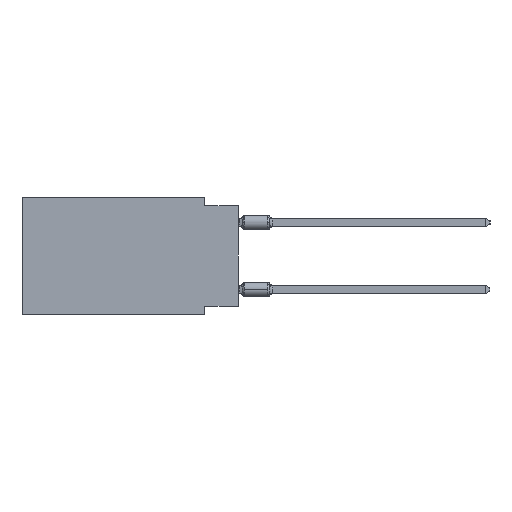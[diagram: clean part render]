
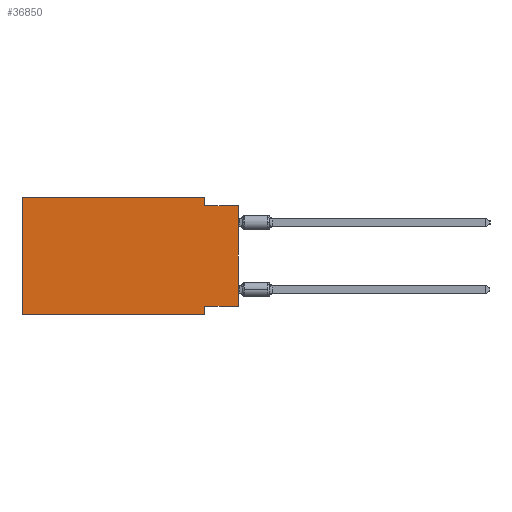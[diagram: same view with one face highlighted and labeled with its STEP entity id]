
A CAD part, left-side view. The second image highlights one B-rep face of the part: STEP entity #36850.
In plain terms, the highlighted planar face has unit normal (-1, 0, 0).
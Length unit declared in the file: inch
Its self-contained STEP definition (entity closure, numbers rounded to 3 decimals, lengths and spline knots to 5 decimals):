
#1203 = CARTESIAN_POINT ( 'NONE',  ( 0., 0., -0.025 ) ) ;
#2034 = ORIENTED_EDGE ( 'NONE', *, *, #37414, .F. ) ;
#2503 = EDGE_CURVE ( 'NONE', #30839, #32852, #24067, .T. ) ;
#3058 = DIRECTION ( 'NONE',  ( 0., -1., 0. ) ) ;
#3201 = EDGE_CURVE ( 'NONE', #14158, #42809, #20255, .T. ) ;
#3870 = DIRECTION ( 'NONE',  ( 0., 0., 1. ) ) ;
#6277 = ORIENTED_EDGE ( 'NONE', *, *, #2503, .F. ) ;
#7036 = VECTOR ( 'NONE', #18807, 39.37008 ) ;
#7081 = EDGE_CURVE ( 'NONE', #27757, #14158, #14231, .T. ) ;
#7306 = LINE ( 'NONE', #21263, #9788 ) ;
#7360 = EDGE_CURVE ( 'NONE', #15903, #43868, #16924, .T. ) ;
#7708 = LINE ( 'NONE', #42487, #31063 ) ;
#9788 = VECTOR ( 'NONE', #3870, 39.37008 ) ;
#9814 = CARTESIAN_POINT ( 'NONE',  ( 0., 0.645, -0.35 ) ) ;
#10117 = FACE_OUTER_BOUND ( 'NONE', #29956, .T. ) ;
#11019 = CARTESIAN_POINT ( 'NONE',  ( 0., 0.1, 0. ) ) ;
#11579 = ORIENTED_EDGE ( 'NONE', *, *, #42791, .F. ) ;
#11835 = EDGE_CURVE ( 'NONE', #30839, #42809, #7708, .T. ) ;
#12063 = CARTESIAN_POINT ( 'NONE',  ( 0., 0.1, 0. ) ) ;
#12819 = AXIS2_PLACEMENT_3D ( 'NONE', #44896, #41465, #17667 ) ;
#13670 = DIRECTION ( 'NONE',  ( 0., 0., 1. ) ) ;
#14158 = VERTEX_POINT ( 'NONE', #15930 ) ;
#14231 = LINE ( 'NONE', #11019, #20646 ) ;
#15883 = VECTOR ( 'NONE', #40990, 39.37008 ) ;
#15903 = VERTEX_POINT ( 'NONE', #40662 ) ;
#15930 = CARTESIAN_POINT ( 'NONE',  ( 0., 0.1, -0.025 ) ) ;
#16818 = CARTESIAN_POINT ( 'NONE',  ( 0., 0., -0.025 ) ) ;
#16907 = VERTEX_POINT ( 'NONE', #29260 ) ;
#16924 = LINE ( 'NONE', #9814, #40402 ) ;
#17667 = DIRECTION ( 'NONE',  ( 0., 0., -1. ) ) ;
#18807 = DIRECTION ( 'NONE',  ( 0., 0., -1. ) ) ;
#20255 = LINE ( 'NONE', #16818, #44344 ) ;
#20548 = ORIENTED_EDGE ( 'NONE', *, *, #3201, .F. ) ;
#20646 = VECTOR ( 'NONE', #38940, 39.37008 ) ;
#21263 = CARTESIAN_POINT ( 'NONE',  ( 0., 0.645, 0. ) ) ;
#21306 = ORIENTED_EDGE ( 'NONE', *, *, #31926, .F. ) ;
#22227 = CARTESIAN_POINT ( 'NONE',  ( 0., 0.1, -0.35 ) ) ;
#23653 = LINE ( 'NONE', #37848, #30740 ) ;
#23673 = DIRECTION ( 'NONE',  ( 0., -1., 0. ) ) ;
#24067 = LINE ( 'NONE', #44435, #15883 ) ;
#25252 = CARTESIAN_POINT ( 'NONE',  ( 0., 0., -0.325 ) ) ;
#27757 = VERTEX_POINT ( 'NONE', #12063 ) ;
#29260 = CARTESIAN_POINT ( 'NONE',  ( 0., 0.645, 0. ) ) ;
#29331 = LINE ( 'NONE', #22227, #7036 ) ;
#29956 = EDGE_LOOP ( 'NONE', ( #34409, #20548, #38769, #21306, #2034, #30920, #11579, #6277 ) ) ;
#30740 = VECTOR ( 'NONE', #3058, 39.37008 ) ;
#30839 = VERTEX_POINT ( 'NONE', #25252 ) ;
#30879 = DIRECTION ( 'NONE',  ( 0., -1., 0. ) ) ;
#30920 = ORIENTED_EDGE ( 'NONE', *, *, #7360, .T. ) ;
#31063 = VECTOR ( 'NONE', #13670, 39.37008 ) ;
#31926 = EDGE_CURVE ( 'NONE', #16907, #27757, #23653, .T. ) ;
#32852 = VERTEX_POINT ( 'NONE', #38861 ) ;
#34409 = ORIENTED_EDGE ( 'NONE', *, *, #11835, .T. ) ;
#36850 = ADVANCED_FACE ( 'NONE', ( #10117 ), #45133, .F. ) ;
#37414 = EDGE_CURVE ( 'NONE', #15903, #16907, #7306, .T. ) ;
#37848 = CARTESIAN_POINT ( 'NONE',  ( 0., 0.645, 0. ) ) ;
#38769 = ORIENTED_EDGE ( 'NONE', *, *, #7081, .F. ) ;
#38861 = CARTESIAN_POINT ( 'NONE',  ( 0., 0.1, -0.325 ) ) ;
#38940 = DIRECTION ( 'NONE',  ( 0., 0., -1. ) ) ;
#40402 = VECTOR ( 'NONE', #30879, 39.37008 ) ;
#40662 = CARTESIAN_POINT ( 'NONE',  ( 0., 0.645, -0.35 ) ) ;
#40990 = DIRECTION ( 'NONE',  ( 0., 1., 0. ) ) ;
#41465 = DIRECTION ( 'NONE',  ( 1., 0., 0. ) ) ;
#41686 = CARTESIAN_POINT ( 'NONE',  ( 0., 0.1, -0.35 ) ) ;
#42487 = CARTESIAN_POINT ( 'NONE',  ( 0., 0., 0. ) ) ;
#42791 = EDGE_CURVE ( 'NONE', #32852, #43868, #29331, .T. ) ;
#42809 = VERTEX_POINT ( 'NONE', #1203 ) ;
#43868 = VERTEX_POINT ( 'NONE', #41686 ) ;
#44344 = VECTOR ( 'NONE', #23673, 39.37008 ) ;
#44435 = CARTESIAN_POINT ( 'NONE',  ( 0., 0., -0.325 ) ) ;
#44896 = CARTESIAN_POINT ( 'NONE',  ( 0., 0.645, 0. ) ) ;
#45133 = PLANE ( 'NONE',  #12819 ) ;
